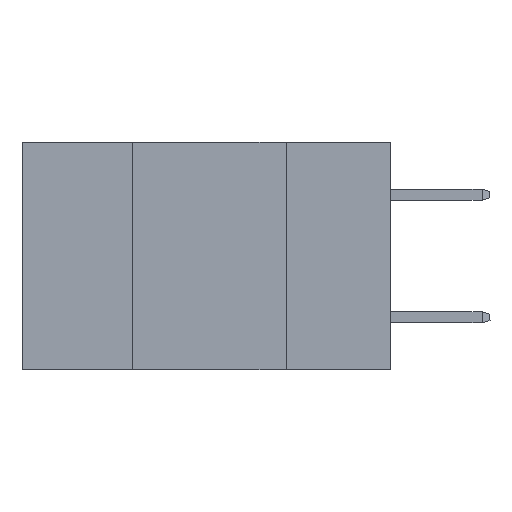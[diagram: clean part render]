
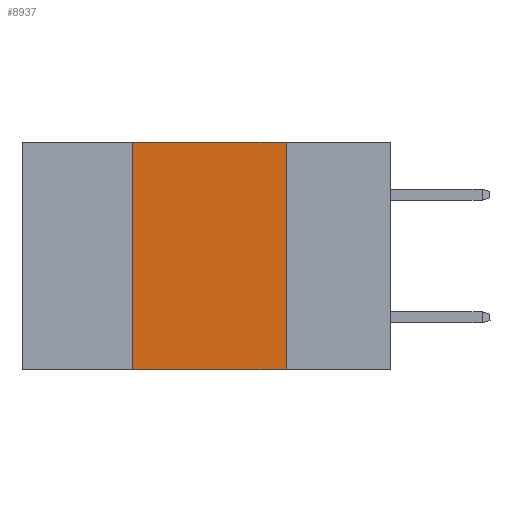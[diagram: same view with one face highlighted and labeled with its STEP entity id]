
A CAD part, left-side view. The second image highlights one B-rep face of the part: STEP entity #8937.
In plain terms, the highlighted planar face has unit normal (-1, 0, 0).
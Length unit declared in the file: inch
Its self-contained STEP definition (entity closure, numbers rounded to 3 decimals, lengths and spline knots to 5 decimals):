
#111 = CARTESIAN_POINT ( 'NONE',  ( 0., 0.17, -0.37 ) ) ;
#141 = FACE_OUTER_BOUND ( 'NONE', #9998, .T. ) ;
#241 = LINE ( 'NONE', #9403, #14570 ) ;
#738 = CARTESIAN_POINT ( 'NONE',  ( 0., 0.17, 0. ) ) ;
#799 = PLANE ( 'NONE',  #3529 ) ;
#914 = LINE ( 'NONE', #738, #15130 ) ;
#2974 = LINE ( 'NONE', #5777, #16777 ) ;
#3006 = CARTESIAN_POINT ( 'NONE',  ( 0., 0.17, 0. ) ) ;
#3529 = AXIS2_PLACEMENT_3D ( 'NONE', #3756, #13334, #5225 ) ;
#3756 = CARTESIAN_POINT ( 'NONE',  ( 0., 0.6, 0. ) ) ;
#3761 = CARTESIAN_POINT ( 'NONE',  ( 0., 0.6, -0.37 ) ) ;
#3805 = ORIENTED_EDGE ( 'NONE', *, *, #17250, .F. ) ;
#4697 = CARTESIAN_POINT ( 'NONE',  ( 0., 0.42, -0.37 ) ) ;
#5225 = DIRECTION ( 'NONE',  ( 0., 0., -1. ) ) ;
#5777 = CARTESIAN_POINT ( 'NONE',  ( 0., 0.42, 0. ) ) ;
#6181 = VERTEX_POINT ( 'NONE', #3006 ) ;
#6574 = EDGE_CURVE ( 'NONE', #16303, #6181, #241, .T. ) ;
#7647 = VERTEX_POINT ( 'NONE', #111 ) ;
#7699 = LINE ( 'NONE', #3761, #11252 ) ;
#7720 = VERTEX_POINT ( 'NONE', #4697 ) ;
#7950 = DIRECTION ( 'NONE',  ( 0., 0., -1. ) ) ;
#8937 = ADVANCED_FACE ( 'NONE', ( #141 ), #799, .F. ) ;
#9224 = EDGE_CURVE ( 'NONE', #7720, #16303, #2974, .T. ) ;
#9403 = CARTESIAN_POINT ( 'NONE',  ( 0., 0.6, 0. ) ) ;
#9945 = DIRECTION ( 'NONE',  ( 0., 0., 1. ) ) ;
#9998 = EDGE_LOOP ( 'NONE', ( #3805, #13841, #11975, #16397 ) ) ;
#11252 = VECTOR ( 'NONE', #17026, 39.37008 ) ;
#11975 = ORIENTED_EDGE ( 'NONE', *, *, #9224, .F. ) ;
#13334 = DIRECTION ( 'NONE',  ( 1., 0., 0. ) ) ;
#13841 = ORIENTED_EDGE ( 'NONE', *, *, #6574, .F. ) ;
#14570 = VECTOR ( 'NONE', #14648, 39.37008 ) ;
#14648 = DIRECTION ( 'NONE',  ( 0., -1., 0. ) ) ;
#15130 = VECTOR ( 'NONE', #7950, 39.37008 ) ;
#16060 = CARTESIAN_POINT ( 'NONE',  ( 0., 0.42, 0. ) ) ;
#16303 = VERTEX_POINT ( 'NONE', #16060 ) ;
#16397 = ORIENTED_EDGE ( 'NONE', *, *, #17272, .T. ) ;
#16777 = VECTOR ( 'NONE', #9945, 39.37008 ) ;
#17026 = DIRECTION ( 'NONE',  ( 0., -1., 0. ) ) ;
#17250 = EDGE_CURVE ( 'NONE', #6181, #7647, #914, .T. ) ;
#17272 = EDGE_CURVE ( 'NONE', #7720, #7647, #7699, .T. ) ;
